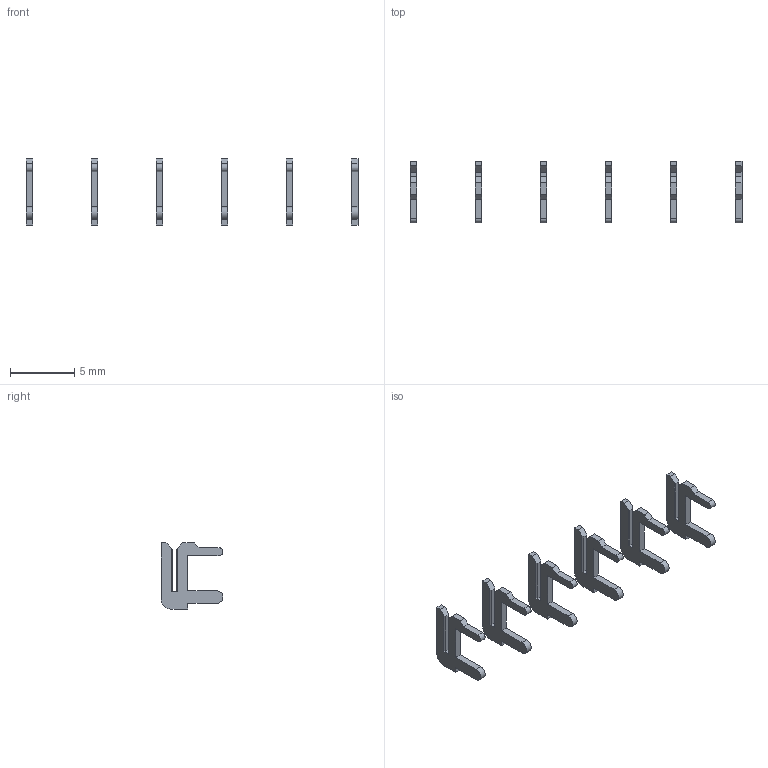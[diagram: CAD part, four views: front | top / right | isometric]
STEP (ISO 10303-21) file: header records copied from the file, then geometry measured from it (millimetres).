
FILE_DESCRIPTION (( 'STEP AP203' ), '1' );
FILE_NAME ('105-006-208-200.STEP', '2020-04-07T22:17:01', ( '' ), ( '' ), 'SwSTEP 2.0', 'SolidWorks 2016', '' );
FILE_SCHEMA (( 'CONFIG_CONTROL_DESIGN' ));
Length unit declared in the file: inch
Products named in the file (2): 100-290-001_100-290-208; 105-006-208-200
Assembly tree (6 placements, depth 2):
  105-006-208-200
    100-290-001_100-290-208  x6
Bounding box: 25.91 x 4.83 x 5.17 mm (x, y, z)
Volume: 41.3 mm3; surface area: 255 mm2
Topology: 6 solids, 6 shells, 150 faces, 414 edges, 276 vertices
Faces by surface type: plane 132, cylinder 18
Entity records: 1149 total; most frequent: CARTESIAN_POINT 149, DIRECTION 143, ORIENTED_EDGE 138, EDGE_CURVE 69, LINE 63, VECTOR 63, VERTEX_POINT 46, AXIS2_PLACEMENT_3D 40
